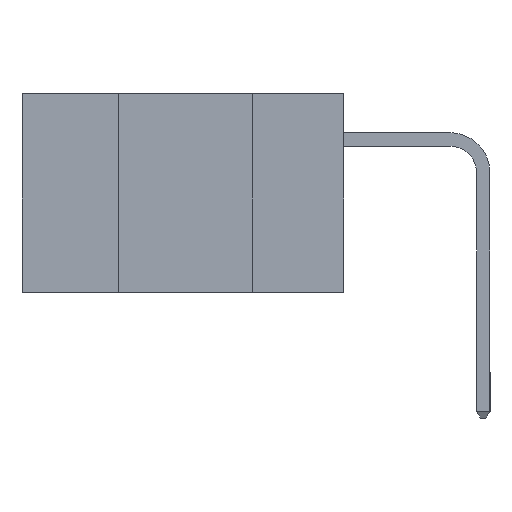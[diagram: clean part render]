
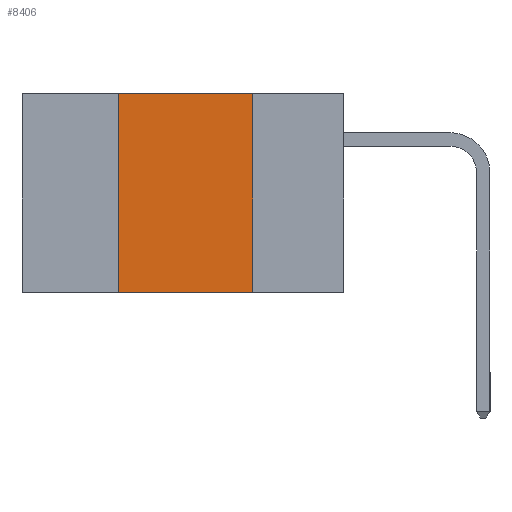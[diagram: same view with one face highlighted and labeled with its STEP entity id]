
A CAD part, left-side view. The second image highlights one B-rep face of the part: STEP entity #8406.
In plain terms, the highlighted planar face has unit normal (-1, 0, 0).
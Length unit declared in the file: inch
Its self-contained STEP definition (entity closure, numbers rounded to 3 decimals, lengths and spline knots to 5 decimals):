
#670 = EDGE_LOOP ( 'NONE', ( #8575, #5802, #7426, #11160 ) ) ;
#800 = DIRECTION ( 'NONE',  ( 0., -1., 0. ) ) ;
#1379 = LINE ( 'NONE', #11098, #2005 ) ;
#2005 = VECTOR ( 'NONE', #10983, 39.37008 ) ;
#2559 = CARTESIAN_POINT ( 'NONE',  ( 0., 0.42, -0.37 ) ) ;
#2692 = CARTESIAN_POINT ( 'NONE',  ( 0., 0.6, -0.37 ) ) ;
#2738 = CARTESIAN_POINT ( 'NONE',  ( 0., 0.6, 0. ) ) ;
#3055 = VERTEX_POINT ( 'NONE', #4127 ) ;
#3222 = LINE ( 'NONE', #10320, #7755 ) ;
#4127 = CARTESIAN_POINT ( 'NONE',  ( 0., 0.17, 0. ) ) ;
#5802 = ORIENTED_EDGE ( 'NONE', *, *, #10963, .F. ) ;
#5828 = DIRECTION ( 'NONE',  ( 0., 0., -1. ) ) ;
#5881 = VERTEX_POINT ( 'NONE', #7072 ) ;
#6132 = CARTESIAN_POINT ( 'NONE',  ( 0., 0.17, -0.37 ) ) ;
#6258 = DIRECTION ( 'NONE',  ( 0., 0., -1. ) ) ;
#6612 = CARTESIAN_POINT ( 'NONE',  ( 0., 0.42, -0.37 ) ) ;
#7072 = CARTESIAN_POINT ( 'NONE',  ( 0., 0.42, 0. ) ) ;
#7134 = FACE_OUTER_BOUND ( 'NONE', #670, .T. ) ;
#7426 = ORIENTED_EDGE ( 'NONE', *, *, #9125, .F. ) ;
#7746 = AXIS2_PLACEMENT_3D ( 'NONE', #2738, #9813, #6258 ) ;
#7755 = VECTOR ( 'NONE', #5828, 39.37008 ) ;
#8406 = ADVANCED_FACE ( 'NONE', ( #7134 ), #10635, .F. ) ;
#8575 = ORIENTED_EDGE ( 'NONE', *, *, #10462, .F. ) ;
#9125 = EDGE_CURVE ( 'NONE', #10952, #5881, #10459, .T. ) ;
#9428 = VECTOR ( 'NONE', #9623, 39.37008 ) ;
#9623 = DIRECTION ( 'NONE',  ( 0., 0., 1. ) ) ;
#9764 = LINE ( 'NONE', #2692, #10852 ) ;
#9813 = DIRECTION ( 'NONE',  ( 1., 0., 0. ) ) ;
#10149 = VERTEX_POINT ( 'NONE', #6132 ) ;
#10320 = CARTESIAN_POINT ( 'NONE',  ( 0., 0.17, -0.37 ) ) ;
#10459 = LINE ( 'NONE', #2559, #9428 ) ;
#10462 = EDGE_CURVE ( 'NONE', #3055, #10149, #3222, .T. ) ;
#10570 = EDGE_CURVE ( 'NONE', #10952, #10149, #9764, .T. ) ;
#10635 = PLANE ( 'NONE',  #7746 ) ;
#10852 = VECTOR ( 'NONE', #800, 39.37008 ) ;
#10952 = VERTEX_POINT ( 'NONE', #6612 ) ;
#10963 = EDGE_CURVE ( 'NONE', #5881, #3055, #1379, .T. ) ;
#10983 = DIRECTION ( 'NONE',  ( 0., -1., 0. ) ) ;
#11098 = CARTESIAN_POINT ( 'NONE',  ( 0., 0.6, 0. ) ) ;
#11160 = ORIENTED_EDGE ( 'NONE', *, *, #10570, .T. ) ;
